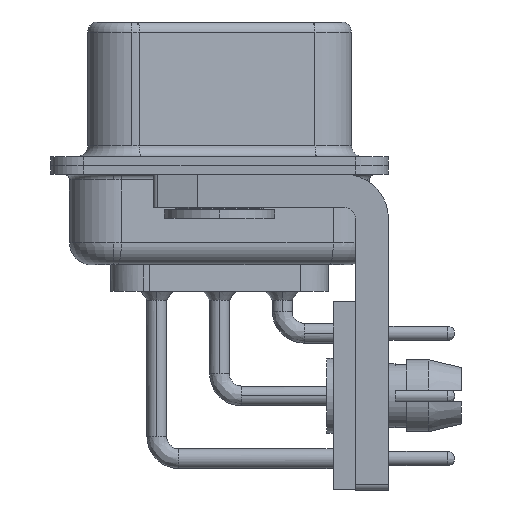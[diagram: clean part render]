
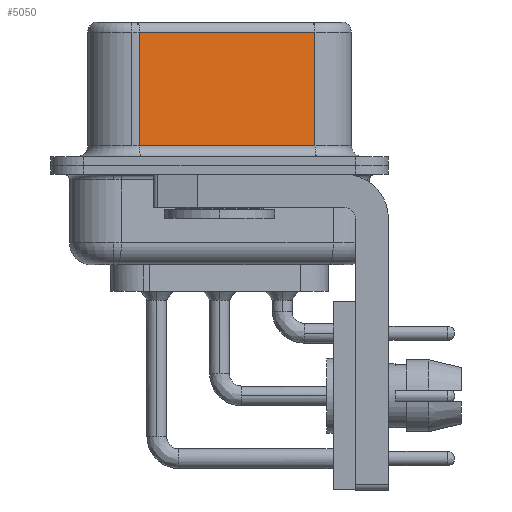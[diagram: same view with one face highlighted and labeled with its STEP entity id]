
A CAD part, left-side view. The second image highlights one B-rep face of the part: STEP entity #5050.
In plain terms, the highlighted planar face has unit normal (-0.985, -0.174, 0).
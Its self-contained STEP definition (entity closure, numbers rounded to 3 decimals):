
#237 = CARTESIAN_POINT ( 'NONE',  ( 3.73, 3.628, 6.02 ) ) ;
#391 = CARTESIAN_POINT ( 'NONE',  ( 3.73, 3.628, 0.9 ) ) ;
#721 = ORIENTED_EDGE ( 'NONE', *, *, #31200, .F. ) ;
#2200 = EDGE_LOOP ( 'NONE', ( #721, #39408, #26547, #28342 ) ) ;
#2910 = VECTOR ( 'NONE', #27887, 1000. ) ;
#3012 = VECTOR ( 'NONE', #27218, 1000. ) ;
#3990 = LINE ( 'NONE', #4274, #2910 ) ;
#4274 = CARTESIAN_POINT ( 'NONE',  ( 3.73, 3.628, 6.52 ) ) ;
#4600 = CARTESIAN_POINT ( 'NONE',  ( 5.132, -4.322, 6.52 ) ) ;
#4717 = EDGE_CURVE ( 'NONE', #22240, #36146, #21642, .T. ) ;
#5050 = ADVANCED_FACE ( 'NONE', ( #43696 ), #8010, .F. ) ;
#6850 = CARTESIAN_POINT ( 'NONE',  ( 5.132, -4.322, 6.52 ) ) ;
#7097 = CARTESIAN_POINT ( 'NONE',  ( 5.132, -4.322, 0.9 ) ) ;
#8010 = PLANE ( 'NONE',  #19211 ) ;
#10874 = VECTOR ( 'NONE', #20717, 1000. ) ;
#11501 = VERTEX_POINT ( 'NONE', #34974 ) ;
#11606 = VECTOR ( 'NONE', #19707, 1000. ) ;
#12031 = LINE ( 'NONE', #6850, #3012 ) ;
#14836 = DIRECTION ( 'NONE',  ( -0.174, 0.985, 0. ) ) ;
#19179 = CARTESIAN_POINT ( 'NONE',  ( 5.132, -4.322, 6.02 ) ) ;
#19211 = AXIS2_PLACEMENT_3D ( 'NONE', #4600, #34966, #14836 ) ;
#19430 = VERTEX_POINT ( 'NONE', #391 ) ;
#19707 = DIRECTION ( 'NONE',  ( -0.174, 0.985, 0. ) ) ;
#19840 = LINE ( 'NONE', #7097, #10874 ) ;
#20717 = DIRECTION ( 'NONE',  ( 0.174, -0.985, 0. ) ) ;
#21642 = LINE ( 'NONE', #32944, #11606 ) ;
#22240 = VERTEX_POINT ( 'NONE', #19179 ) ;
#26547 = ORIENTED_EDGE ( 'NONE', *, *, #39667, .T. ) ;
#27218 = DIRECTION ( 'NONE',  ( 0., 0., -1. ) ) ;
#27887 = DIRECTION ( 'NONE',  ( 0., 0., -1. ) ) ;
#28342 = ORIENTED_EDGE ( 'NONE', *, *, #32209, .T. ) ;
#31200 = EDGE_CURVE ( 'NONE', #22240, #11501, #12031, .T. ) ;
#32209 = EDGE_CURVE ( 'NONE', #19430, #11501, #19840, .T. ) ;
#32944 = CARTESIAN_POINT ( 'NONE',  ( 5.132, -4.322, 6.02 ) ) ;
#34966 = DIRECTION ( 'NONE',  ( 0.985, 0.174, 0. ) ) ;
#34974 = CARTESIAN_POINT ( 'NONE',  ( 5.132, -4.322, 0.9 ) ) ;
#36146 = VERTEX_POINT ( 'NONE', #237 ) ;
#39408 = ORIENTED_EDGE ( 'NONE', *, *, #4717, .T. ) ;
#39667 = EDGE_CURVE ( 'NONE', #36146, #19430, #3990, .T. ) ;
#43696 = FACE_OUTER_BOUND ( 'NONE', #2200, .T. ) ;
